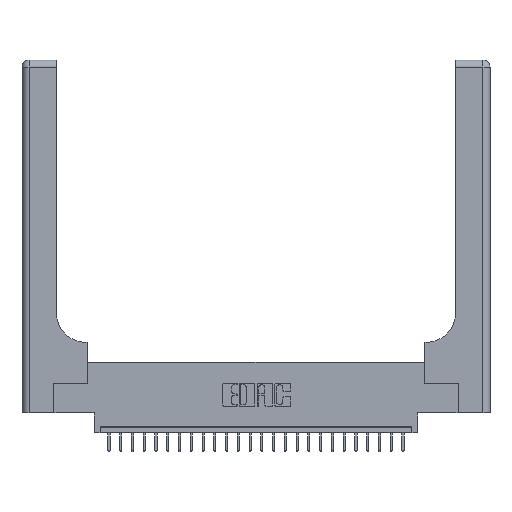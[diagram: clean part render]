
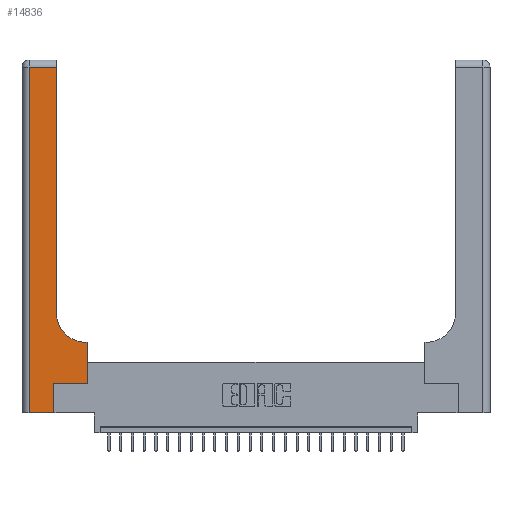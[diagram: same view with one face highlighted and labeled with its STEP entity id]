
A CAD part, top view. The second image highlights one B-rep face of the part: STEP entity #14836.
In plain terms, the highlighted planar face has unit normal (0, 0, 1).
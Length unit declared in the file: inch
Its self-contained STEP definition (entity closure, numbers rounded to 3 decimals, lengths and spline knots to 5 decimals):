
#15 = CARTESIAN_POINT ( 'NONE',  ( 0.06, 2.94, 0.37 ) ) ;
#722 = LINE ( 'NONE', #4751, #12528 ) ;
#838 = CARTESIAN_POINT ( 'NONE',  ( 0.5585, 0.25, 0.37 ) ) ;
#1105 = EDGE_CURVE ( 'NONE', #24737, #14097, #8363, .T. ) ;
#1121 = ORIENTED_EDGE ( 'NONE', *, *, #12163, .T. ) ;
#2151 = AXIS2_PLACEMENT_3D ( 'NONE', #9375, #15784, #11323 ) ;
#2672 = CARTESIAN_POINT ( 'NONE',  ( 0.5415, 0.85, 0.37 ) ) ;
#3042 = DIRECTION ( 'NONE',  ( -1., 0., 0. ) ) ;
#3713 = ORIENTED_EDGE ( 'NONE', *, *, #26902, .T. ) ;
#3766 = ORIENTED_EDGE ( 'NONE', *, *, #20673, .T. ) ;
#3811 = VECTOR ( 'NONE', #21114, 39.37008 ) ;
#3981 = ORIENTED_EDGE ( 'NONE', *, *, #18255, .T. ) ;
#4263 = EDGE_CURVE ( 'NONE', #16712, #5119, #20235, .T. ) ;
#4357 = VERTEX_POINT ( 'NONE', #17029 ) ;
#4521 = FACE_OUTER_BOUND ( 'NONE', #17679, .T. ) ;
#4751 = CARTESIAN_POINT ( 'NONE',  ( 0.5585, 0.25, 0.37 ) ) ;
#4842 = CARTESIAN_POINT ( 'NONE',  ( 0.269, 0., 0.37 ) ) ;
#5119 = VERTEX_POINT ( 'NONE', #16637 ) ;
#5520 = ORIENTED_EDGE ( 'NONE', *, *, #1105, .T. ) ;
#5540 = DIRECTION ( 'NONE',  ( 0., -1., 0. ) ) ;
#6047 = VERTEX_POINT ( 'NONE', #4842 ) ;
#6652 = VECTOR ( 'NONE', #3042, 39.37008 ) ;
#6666 = DIRECTION ( 'NONE',  ( 0., 1., 0. ) ) ;
#7531 = LINE ( 'NONE', #9452, #18022 ) ;
#7876 = VERTEX_POINT ( 'NONE', #19118 ) ;
#8057 = VECTOR ( 'NONE', #16257, 39.37008 ) ;
#8295 = EDGE_CURVE ( 'NONE', #11677, #24737, #23319, .T. ) ;
#8363 = CIRCLE ( 'NONE', #24242, 0.25 ) ;
#8505 = CARTESIAN_POINT ( 'NONE',  ( 0., 2.94, 0.37 ) ) ;
#9020 = VECTOR ( 'NONE', #13678, 39.37008 ) ;
#9375 = CARTESIAN_POINT ( 'NONE',  ( 0., 3., 0.37 ) ) ;
#9452 = CARTESIAN_POINT ( 'NONE',  ( 0.2915, 3., 0.37 ) ) ;
#11323 = DIRECTION ( 'NONE',  ( -1., 0., 0. ) ) ;
#11677 = VERTEX_POINT ( 'NONE', #17308 ) ;
#12163 = EDGE_CURVE ( 'NONE', #14751, #11677, #722, .T. ) ;
#12424 = ORIENTED_EDGE ( 'NONE', *, *, #24841, .T. ) ;
#12528 = VECTOR ( 'NONE', #6666, 39.37008 ) ;
#12815 = ORIENTED_EDGE ( 'NONE', *, *, #8295, .T. ) ;
#13261 = LINE ( 'NONE', #17533, #9020 ) ;
#13335 = CARTESIAN_POINT ( 'NONE',  ( 0.2915, 0.85, 0.37 ) ) ;
#13678 = DIRECTION ( 'NONE',  ( 1., 0., 0. ) ) ;
#14097 = VERTEX_POINT ( 'NONE', #13335 ) ;
#14751 = VERTEX_POINT ( 'NONE', #838 ) ;
#14836 = ADVANCED_FACE ( 'NONE', ( #4521 ), #17613, .F. ) ;
#15784 = DIRECTION ( 'NONE',  ( 0., 0., -1. ) ) ;
#15917 = LINE ( 'NONE', #8505, #3811 ) ;
#16257 = DIRECTION ( 'NONE',  ( 1., 0., 0. ) ) ;
#16528 = CARTESIAN_POINT ( 'NONE',  ( 0.269, 0.25, 0.37 ) ) ;
#16637 = CARTESIAN_POINT ( 'NONE',  ( 0.06, 0., 0.37 ) ) ;
#16712 = VERTEX_POINT ( 'NONE', #15 ) ;
#17029 = CARTESIAN_POINT ( 'NONE',  ( 0.269, 0.25, 0.37 ) ) ;
#17308 = CARTESIAN_POINT ( 'NONE',  ( 0.5585, 0.6, 0.37 ) ) ;
#17500 = CARTESIAN_POINT ( 'NONE',  ( 0.269, 0., 0.37 ) ) ;
#17533 = CARTESIAN_POINT ( 'NONE',  ( 0., 0., 0.37 ) ) ;
#17613 = PLANE ( 'NONE',  #2151 ) ;
#17679 = EDGE_LOOP ( 'NONE', ( #12424, #3713, #22211, #22021, #3981, #3766, #1121, #12815, #5520 ) ) ;
#17794 = CARTESIAN_POINT ( 'NONE',  ( 0.2915, 0.6, 0.37 ) ) ;
#18022 = VECTOR ( 'NONE', #26354, 39.37008 ) ;
#18109 = CARTESIAN_POINT ( 'NONE',  ( 0.06, 3., 0.37 ) ) ;
#18255 = EDGE_CURVE ( 'NONE', #6047, #4357, #21272, .T. ) ;
#18932 = VECTOR ( 'NONE', #5540, 39.37008 ) ;
#19118 = CARTESIAN_POINT ( 'NONE',  ( 0.2915, 2.94, 0.37 ) ) ;
#19417 = DIRECTION ( 'NONE',  ( 0., 1., 0. ) ) ;
#20235 = LINE ( 'NONE', #18109, #18932 ) ;
#20673 = EDGE_CURVE ( 'NONE', #4357, #14751, #24059, .T. ) ;
#21032 = EDGE_CURVE ( 'NONE', #5119, #6047, #13261, .T. ) ;
#21114 = DIRECTION ( 'NONE',  ( -1., 0., 0. ) ) ;
#21138 = DIRECTION ( 'NONE',  ( 1., 0., 0. ) ) ;
#21272 = LINE ( 'NONE', #17500, #26204 ) ;
#22021 = ORIENTED_EDGE ( 'NONE', *, *, #21032, .T. ) ;
#22211 = ORIENTED_EDGE ( 'NONE', *, *, #4263, .T. ) ;
#23319 = LINE ( 'NONE', #17794, #6652 ) ;
#24059 = LINE ( 'NONE', #16528, #8057 ) ;
#24242 = AXIS2_PLACEMENT_3D ( 'NONE', #2672, #25224, #21138 ) ;
#24737 = VERTEX_POINT ( 'NONE', #25967 ) ;
#24841 = EDGE_CURVE ( 'NONE', #14097, #7876, #7531, .T. ) ;
#25224 = DIRECTION ( 'NONE',  ( 0., 0., -1. ) ) ;
#25967 = CARTESIAN_POINT ( 'NONE',  ( 0.5415, 0.6, 0.37 ) ) ;
#26204 = VECTOR ( 'NONE', #19417, 39.37008 ) ;
#26354 = DIRECTION ( 'NONE',  ( 0., 1., 0. ) ) ;
#26902 = EDGE_CURVE ( 'NONE', #7876, #16712, #15917, .T. ) ;
